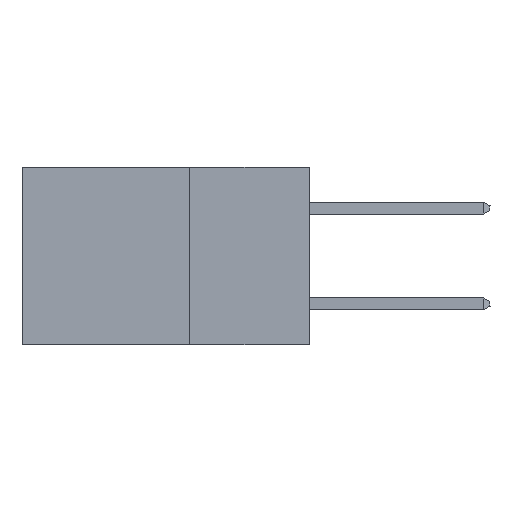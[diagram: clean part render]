
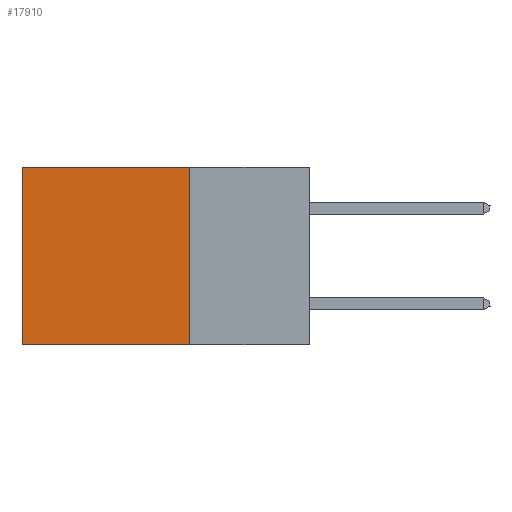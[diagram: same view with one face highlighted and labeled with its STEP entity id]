
A CAD part, left-side view. The second image highlights one B-rep face of the part: STEP entity #17910.
In plain terms, the highlighted planar face has unit normal (-1, 0, 0).
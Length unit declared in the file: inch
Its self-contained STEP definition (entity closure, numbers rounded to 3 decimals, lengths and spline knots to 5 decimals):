
#213 = VERTEX_POINT ( 'NONE', #6228 ) ;
#638 = CARTESIAN_POINT ( 'NONE',  ( 0.2875, 0.6, -0.37 ) ) ;
#676 = EDGE_LOOP ( 'NONE', ( #14794, #11816, #15852, #6947 ) ) ;
#705 = PLANE ( 'NONE',  #10008 ) ;
#769 = EDGE_CURVE ( 'NONE', #18219, #17975, #11702, .T. ) ;
#772 = LINE ( 'NONE', #13557, #17830 ) ;
#2312 = DIRECTION ( 'NONE',  ( 1., 0., 0. ) ) ;
#2814 = FACE_OUTER_BOUND ( 'NONE', #676, .T. ) ;
#3127 = EDGE_CURVE ( 'NONE', #213, #18219, #772, .T. ) ;
#6228 = CARTESIAN_POINT ( 'NONE',  ( 0.2875, 0.25, 0. ) ) ;
#6233 = LINE ( 'NONE', #18472, #14214 ) ;
#6947 = ORIENTED_EDGE ( 'NONE', *, *, #3127, .T. ) ;
#9018 = DIRECTION ( 'NONE',  ( 0., 0., -1. ) ) ;
#9259 = VECTOR ( 'NONE', #9018, 39.37008 ) ;
#9949 = VERTEX_POINT ( 'NONE', #16606 ) ;
#10008 = AXIS2_PLACEMENT_3D ( 'NONE', #13041, #2312, #11349 ) ;
#11349 = DIRECTION ( 'NONE',  ( 0., 0., -1. ) ) ;
#11702 = LINE ( 'NONE', #11977, #17412 ) ;
#11816 = ORIENTED_EDGE ( 'NONE', *, *, #16109, .F. ) ;
#11906 = LINE ( 'NONE', #18200, #9259 ) ;
#11977 = CARTESIAN_POINT ( 'NONE',  ( 0.2875, 0.6, 0. ) ) ;
#13041 = CARTESIAN_POINT ( 'NONE',  ( 0.2875, 0.25, 0. ) ) ;
#13286 = DIRECTION ( 'NONE',  ( 0., 1., 0. ) ) ;
#13557 = CARTESIAN_POINT ( 'NONE',  ( 0.2875, 0.25, 0. ) ) ;
#14214 = VECTOR ( 'NONE', #18282, 39.37008 ) ;
#14794 = ORIENTED_EDGE ( 'NONE', *, *, #769, .T. ) ;
#15852 = ORIENTED_EDGE ( 'NONE', *, *, #19528, .F. ) ;
#16109 = EDGE_CURVE ( 'NONE', #9949, #17975, #6233, .T. ) ;
#16293 = DIRECTION ( 'NONE',  ( 0., 0., -1. ) ) ;
#16606 = CARTESIAN_POINT ( 'NONE',  ( 0.2875, 0.25, -0.37 ) ) ;
#17412 = VECTOR ( 'NONE', #16293, 39.37008 ) ;
#17830 = VECTOR ( 'NONE', #13286, 39.37008 ) ;
#17910 = ADVANCED_FACE ( 'NONE', ( #2814 ), #705, .F. ) ;
#17975 = VERTEX_POINT ( 'NONE', #638 ) ;
#18200 = CARTESIAN_POINT ( 'NONE',  ( 0.2875, 0.25, 0. ) ) ;
#18219 = VERTEX_POINT ( 'NONE', #18445 ) ;
#18282 = DIRECTION ( 'NONE',  ( 0., 1., 0. ) ) ;
#18445 = CARTESIAN_POINT ( 'NONE',  ( 0.2875, 0.6, 0. ) ) ;
#18472 = CARTESIAN_POINT ( 'NONE',  ( 0.2875, 0.25, -0.37 ) ) ;
#19528 = EDGE_CURVE ( 'NONE', #213, #9949, #11906, .T. ) ;
